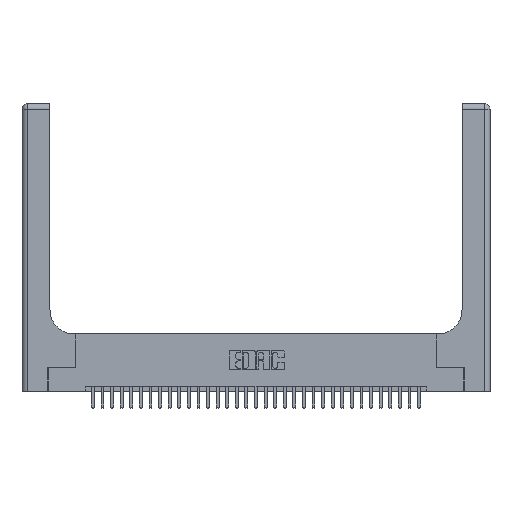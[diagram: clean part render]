
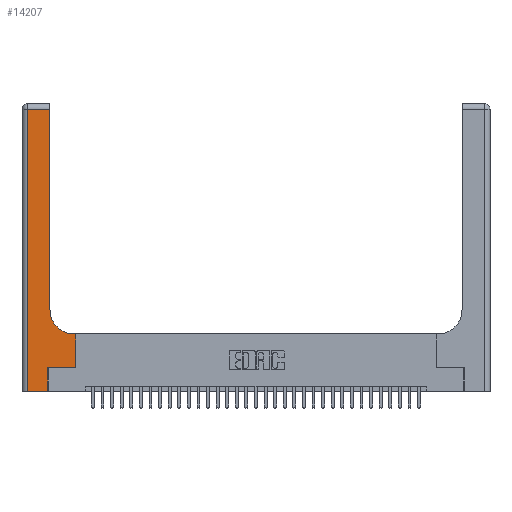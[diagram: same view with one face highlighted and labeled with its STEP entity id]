
A CAD part, top view. The second image highlights one B-rep face of the part: STEP entity #14207.
In plain terms, the highlighted planar face has unit normal (0, 0, 1).
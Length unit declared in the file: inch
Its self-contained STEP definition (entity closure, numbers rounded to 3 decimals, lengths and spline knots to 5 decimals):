
#49 = DIRECTION ( 'NONE',  ( 0., 1., 0. ) ) ;
#127 = EDGE_CURVE ( 'NONE', #19977, #672, #18551, .T. ) ;
#672 = VERTEX_POINT ( 'NONE', #18278 ) ;
#950 = FACE_OUTER_BOUND ( 'NONE', #32164, .T. ) ;
#1206 = LINE ( 'NONE', #8663, #27718 ) ;
#1628 = EDGE_CURVE ( 'NONE', #15290, #29291, #16007, .T. ) ;
#2456 = CARTESIAN_POINT ( 'NONE',  ( 0.269, 0.25, 0.37 ) ) ;
#2575 = DIRECTION ( 'NONE',  ( 0., 0., -1. ) ) ;
#2952 = EDGE_CURVE ( 'NONE', #15927, #3903, #10291, .T. ) ;
#3218 = ORIENTED_EDGE ( 'NONE', *, *, #18506, .T. ) ;
#3903 = VERTEX_POINT ( 'NONE', #6887 ) ;
#4078 = VECTOR ( 'NONE', #27057, 39.37008 ) ;
#4695 = LINE ( 'NONE', #13175, #21334 ) ;
#4841 = CARTESIAN_POINT ( 'NONE',  ( 0.269, 0.25, 0.37 ) ) ;
#4963 = CARTESIAN_POINT ( 'NONE',  ( 0.06, 0., 0.37 ) ) ;
#6220 = DIRECTION ( 'NONE',  ( 0., 1., 0. ) ) ;
#6887 = CARTESIAN_POINT ( 'NONE',  ( 0.2915, 0.85, 0.37 ) ) ;
#6996 = VECTOR ( 'NONE', #6220, 39.37008 ) ;
#7537 = CARTESIAN_POINT ( 'NONE',  ( 0.5415, 0.6, 0.37 ) ) ;
#8559 = DIRECTION ( 'NONE',  ( 1., 0., 0. ) ) ;
#8663 = CARTESIAN_POINT ( 'NONE',  ( 0.5585, 0.25, 0.37 ) ) ;
#8755 = EDGE_CURVE ( 'NONE', #672, #23559, #1206, .T. ) ;
#8871 = CARTESIAN_POINT ( 'NONE',  ( 0., 2.94, 0.37 ) ) ;
#9128 = DIRECTION ( 'NONE',  ( -1., 0., 0. ) ) ;
#9907 = DIRECTION ( 'NONE',  ( 0., -1., 0. ) ) ;
#10291 = CIRCLE ( 'NONE', #13046, 0.25 ) ;
#10839 = CARTESIAN_POINT ( 'NONE',  ( 0.5585, 0.6, 0.37 ) ) ;
#11655 = VECTOR ( 'NONE', #19946, 39.37008 ) ;
#12958 = LINE ( 'NONE', #21929, #28413 ) ;
#13046 = AXIS2_PLACEMENT_3D ( 'NONE', #21126, #28973, #31369 ) ;
#13175 = CARTESIAN_POINT ( 'NONE',  ( 0.269, 0., 0.37 ) ) ;
#13532 = ORIENTED_EDGE ( 'NONE', *, *, #127, .T. ) ;
#13857 = ORIENTED_EDGE ( 'NONE', *, *, #26662, .T. ) ;
#14207 = ADVANCED_FACE ( 'NONE', ( #950 ), #31175, .F. ) ;
#14364 = ORIENTED_EDGE ( 'NONE', *, *, #2952, .T. ) ;
#14414 = CARTESIAN_POINT ( 'NONE',  ( 0.2915, 3., 0.37 ) ) ;
#15290 = VERTEX_POINT ( 'NONE', #4963 ) ;
#15618 = CARTESIAN_POINT ( 'NONE',  ( 0., 3., 0.37 ) ) ;
#15927 = VERTEX_POINT ( 'NONE', #7537 ) ;
#16007 = LINE ( 'NONE', #18677, #27411 ) ;
#16457 = EDGE_CURVE ( 'NONE', #30507, #15290, #33356, .T. ) ;
#17862 = ORIENTED_EDGE ( 'NONE', *, *, #23905, .T. ) ;
#18229 = DIRECTION ( 'NONE',  ( -1., 0., 0. ) ) ;
#18278 = CARTESIAN_POINT ( 'NONE',  ( 0.5585, 0.25, 0.37 ) ) ;
#18506 = EDGE_CURVE ( 'NONE', #3903, #33201, #28570, .T. ) ;
#18551 = LINE ( 'NONE', #4841, #11655 ) ;
#18677 = CARTESIAN_POINT ( 'NONE',  ( 0., 0., 0.37 ) ) ;
#19543 = AXIS2_PLACEMENT_3D ( 'NONE', #15618, #2575, #18229 ) ;
#19946 = DIRECTION ( 'NONE',  ( 1., 0., 0. ) ) ;
#19977 = VERTEX_POINT ( 'NONE', #2456 ) ;
#20006 = CARTESIAN_POINT ( 'NONE',  ( 0.06, 3., 0.37 ) ) ;
#20976 = EDGE_CURVE ( 'NONE', #23559, #15927, #12958, .T. ) ;
#21126 = CARTESIAN_POINT ( 'NONE',  ( 0.5415, 0.85, 0.37 ) ) ;
#21334 = VECTOR ( 'NONE', #49, 39.37008 ) ;
#21929 = CARTESIAN_POINT ( 'NONE',  ( 0.2915, 0.6, 0.37 ) ) ;
#22343 = ORIENTED_EDGE ( 'NONE', *, *, #16457, .T. ) ;
#23559 = VERTEX_POINT ( 'NONE', #10839 ) ;
#23905 = EDGE_CURVE ( 'NONE', #29291, #19977, #4695, .T. ) ;
#23994 = CARTESIAN_POINT ( 'NONE',  ( 0.06, 2.94, 0.37 ) ) ;
#26662 = EDGE_CURVE ( 'NONE', #33201, #30507, #28094, .T. ) ;
#27057 = DIRECTION ( 'NONE',  ( -1., 0., 0. ) ) ;
#27250 = ORIENTED_EDGE ( 'NONE', *, *, #8755, .T. ) ;
#27411 = VECTOR ( 'NONE', #8559, 39.37008 ) ;
#27718 = VECTOR ( 'NONE', #29237, 39.37008 ) ;
#28094 = LINE ( 'NONE', #8871, #4078 ) ;
#28101 = VECTOR ( 'NONE', #9907, 39.37008 ) ;
#28413 = VECTOR ( 'NONE', #9128, 39.37008 ) ;
#28436 = CARTESIAN_POINT ( 'NONE',  ( 0.269, 0., 0.37 ) ) ;
#28570 = LINE ( 'NONE', #14414, #6996 ) ;
#28588 = CARTESIAN_POINT ( 'NONE',  ( 0.2915, 2.94, 0.37 ) ) ;
#28973 = DIRECTION ( 'NONE',  ( 0., 0., -1. ) ) ;
#29237 = DIRECTION ( 'NONE',  ( 0., 1., 0. ) ) ;
#29291 = VERTEX_POINT ( 'NONE', #28436 ) ;
#30507 = VERTEX_POINT ( 'NONE', #23994 ) ;
#31175 = PLANE ( 'NONE',  #19543 ) ;
#31369 = DIRECTION ( 'NONE',  ( 1., 0., 0. ) ) ;
#32164 = EDGE_LOOP ( 'NONE', ( #3218, #13857, #22343, #32659, #17862, #13532, #27250, #32515, #14364 ) ) ;
#32515 = ORIENTED_EDGE ( 'NONE', *, *, #20976, .T. ) ;
#32659 = ORIENTED_EDGE ( 'NONE', *, *, #1628, .T. ) ;
#33201 = VERTEX_POINT ( 'NONE', #28588 ) ;
#33356 = LINE ( 'NONE', #20006, #28101 ) ;
